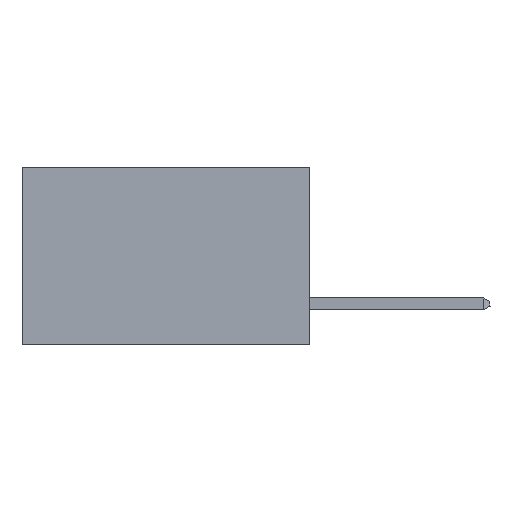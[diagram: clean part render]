
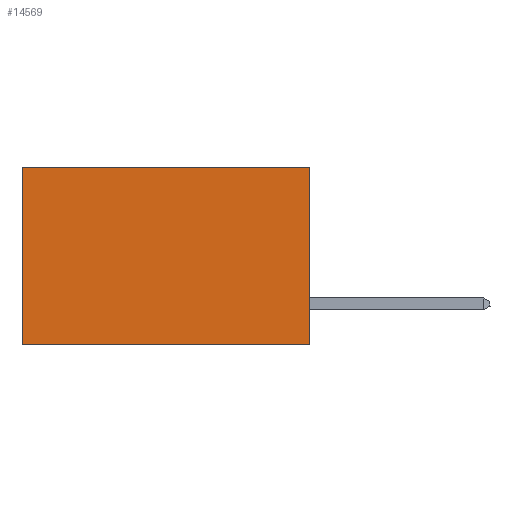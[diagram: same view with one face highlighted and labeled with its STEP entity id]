
A CAD part, left-side view. The second image highlights one B-rep face of the part: STEP entity #14569.
In plain terms, the highlighted planar face has unit normal (-1, 0, 0).
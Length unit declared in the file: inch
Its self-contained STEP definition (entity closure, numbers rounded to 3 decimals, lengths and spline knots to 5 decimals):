
#435 = VECTOR ( 'NONE', #30999, 39.37008 ) ;
#922 = EDGE_CURVE ( 'NONE', #3219, #34631, #21302, .T. ) ;
#1175 = AXIS2_PLACEMENT_3D ( 'NONE', #4879, #41482, #15900 ) ;
#3219 = VERTEX_POINT ( 'NONE', #43418 ) ;
#3583 = EDGE_CURVE ( 'NONE', #46045, #28850, #18088, .T. ) ;
#3990 = LINE ( 'NONE', #27366, #42020 ) ;
#4879 = CARTESIAN_POINT ( 'NONE',  ( 0.2875, 0., 0. ) ) ;
#6390 = CARTESIAN_POINT ( 'NONE',  ( 0.2875, 0.6, 0. ) ) ;
#8093 = VECTOR ( 'NONE', #18082, 39.37008 ) ;
#9809 = LINE ( 'NONE', #11570, #12067 ) ;
#11076 = ORIENTED_EDGE ( 'NONE', *, *, #27775, .T. ) ;
#11570 = CARTESIAN_POINT ( 'NONE',  ( 0.2875, 0., 0. ) ) ;
#12067 = VECTOR ( 'NONE', #22704, 39.37008 ) ;
#13561 = ORIENTED_EDGE ( 'NONE', *, *, #922, .F. ) ;
#13932 = CARTESIAN_POINT ( 'NONE',  ( 0.2875, 0., 0. ) ) ;
#14569 = ADVANCED_FACE ( 'NONE', ( #46571 ), #34236, .F. ) ;
#15008 = CARTESIAN_POINT ( 'NONE',  ( 0.2875, 0.6, -0.37 ) ) ;
#15900 = DIRECTION ( 'NONE',  ( 0., 0., -1. ) ) ;
#18082 = DIRECTION ( 'NONE',  ( 0., 1., 0. ) ) ;
#18088 = LINE ( 'NONE', #34435, #435 ) ;
#21302 = LINE ( 'NONE', #46755, #8093 ) ;
#22704 = DIRECTION ( 'NONE',  ( 0., 0., -1. ) ) ;
#23349 = EDGE_LOOP ( 'NONE', ( #11076, #13561, #33004, #26518 ) ) ;
#26518 = ORIENTED_EDGE ( 'NONE', *, *, #3583, .T. ) ;
#27366 = CARTESIAN_POINT ( 'NONE',  ( 0.2875, 0.6, 0. ) ) ;
#27775 = EDGE_CURVE ( 'NONE', #28850, #34631, #3990, .T. ) ;
#28850 = VERTEX_POINT ( 'NONE', #6390 ) ;
#30999 = DIRECTION ( 'NONE',  ( 0., 1., 0. ) ) ;
#33004 = ORIENTED_EDGE ( 'NONE', *, *, #40424, .F. ) ;
#34236 = PLANE ( 'NONE',  #1175 ) ;
#34435 = CARTESIAN_POINT ( 'NONE',  ( 0.2875, 0., 0. ) ) ;
#34631 = VERTEX_POINT ( 'NONE', #15008 ) ;
#38222 = DIRECTION ( 'NONE',  ( 0., 0., -1. ) ) ;
#40424 = EDGE_CURVE ( 'NONE', #46045, #3219, #9809, .T. ) ;
#41482 = DIRECTION ( 'NONE',  ( 1., 0., 0. ) ) ;
#42020 = VECTOR ( 'NONE', #38222, 39.37008 ) ;
#43418 = CARTESIAN_POINT ( 'NONE',  ( 0.2875, 0., -0.37 ) ) ;
#46045 = VERTEX_POINT ( 'NONE', #13932 ) ;
#46571 = FACE_OUTER_BOUND ( 'NONE', #23349, .T. ) ;
#46755 = CARTESIAN_POINT ( 'NONE',  ( 0.2875, 0., -0.37 ) ) ;
